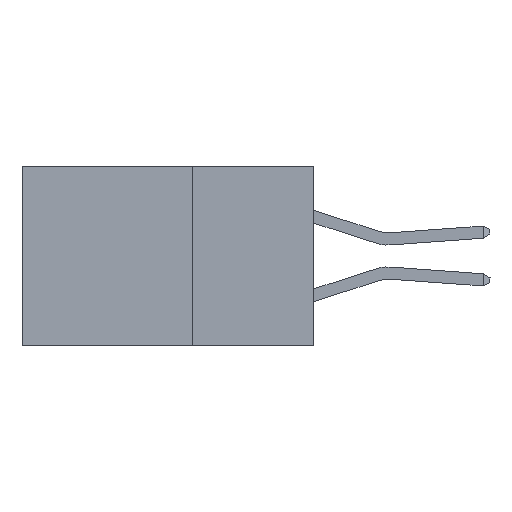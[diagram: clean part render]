
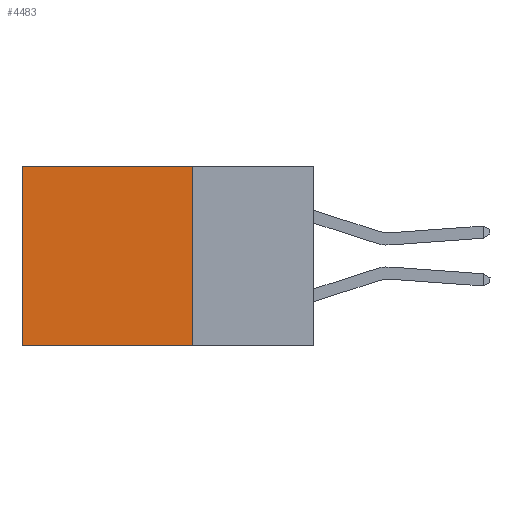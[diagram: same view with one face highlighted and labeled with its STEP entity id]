
A CAD part, left-side view. The second image highlights one B-rep face of the part: STEP entity #4483.
In plain terms, the highlighted planar face has unit normal (-1, 0, 0).
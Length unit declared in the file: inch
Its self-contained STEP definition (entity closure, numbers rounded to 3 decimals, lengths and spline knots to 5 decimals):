
#1183 = ORIENTED_EDGE ( 'NONE', *, *, #15447, .F. ) ;
#1285 = CARTESIAN_POINT ( 'NONE',  ( 0.2875, 0.6, 0. ) ) ;
#1613 = FACE_OUTER_BOUND ( 'NONE', #13892, .T. ) ;
#1759 = EDGE_CURVE ( 'NONE', #12997, #11319, #10382, .T. ) ;
#2757 = PLANE ( 'NONE',  #9415 ) ;
#3682 = DIRECTION ( 'NONE',  ( 1., 0., 0. ) ) ;
#3928 = LINE ( 'NONE', #17209, #13202 ) ;
#4483 = ADVANCED_FACE ( 'NONE', ( #1613 ), #2757, .F. ) ;
#5644 = CARTESIAN_POINT ( 'NONE',  ( 0.2875, 0.25, -0.37 ) ) ;
#7065 = CARTESIAN_POINT ( 'NONE',  ( 0.2875, 0.25, 0. ) ) ;
#8077 = DIRECTION ( 'NONE',  ( 0., 0., -1. ) ) ;
#8732 = EDGE_CURVE ( 'NONE', #15300, #20946, #3928, .T. ) ;
#8984 = VECTOR ( 'NONE', #19041, 39.37008 ) ;
#9415 = AXIS2_PLACEMENT_3D ( 'NONE', #20966, #3682, #11164 ) ;
#9807 = CARTESIAN_POINT ( 'NONE',  ( 0.2875, 0.25, -0.37 ) ) ;
#10382 = LINE ( 'NONE', #1285, #8984 ) ;
#10984 = VECTOR ( 'NONE', #18843, 39.37008 ) ;
#11021 = ORIENTED_EDGE ( 'NONE', *, *, #8732, .F. ) ;
#11164 = DIRECTION ( 'NONE',  ( 0., 0., -1. ) ) ;
#11319 = VERTEX_POINT ( 'NONE', #11820 ) ;
#11490 = EDGE_CURVE ( 'NONE', #15300, #12997, #20165, .T. ) ;
#11820 = CARTESIAN_POINT ( 'NONE',  ( 0.2875, 0.6, -0.37 ) ) ;
#12997 = VERTEX_POINT ( 'NONE', #18377 ) ;
#13202 = VECTOR ( 'NONE', #8077, 39.37008 ) ;
#13892 = EDGE_LOOP ( 'NONE', ( #19153, #1183, #11021, #20863 ) ) ;
#15300 = VERTEX_POINT ( 'NONE', #7065 ) ;
#15447 = EDGE_CURVE ( 'NONE', #20946, #11319, #18062, .T. ) ;
#17209 = CARTESIAN_POINT ( 'NONE',  ( 0.2875, 0.25, 0. ) ) ;
#17658 = VECTOR ( 'NONE', #23278, 39.37008 ) ;
#18062 = LINE ( 'NONE', #9807, #10984 ) ;
#18377 = CARTESIAN_POINT ( 'NONE',  ( 0.2875, 0.6, 0. ) ) ;
#18843 = DIRECTION ( 'NONE',  ( 0., 1., 0. ) ) ;
#19041 = DIRECTION ( 'NONE',  ( 0., 0., -1. ) ) ;
#19153 = ORIENTED_EDGE ( 'NONE', *, *, #1759, .T. ) ;
#19618 = CARTESIAN_POINT ( 'NONE',  ( 0.2875, 0.25, 0. ) ) ;
#20165 = LINE ( 'NONE', #19618, #17658 ) ;
#20863 = ORIENTED_EDGE ( 'NONE', *, *, #11490, .T. ) ;
#20946 = VERTEX_POINT ( 'NONE', #5644 ) ;
#20966 = CARTESIAN_POINT ( 'NONE',  ( 0.2875, 0.25, 0. ) ) ;
#23278 = DIRECTION ( 'NONE',  ( 0., 1., 0. ) ) ;
